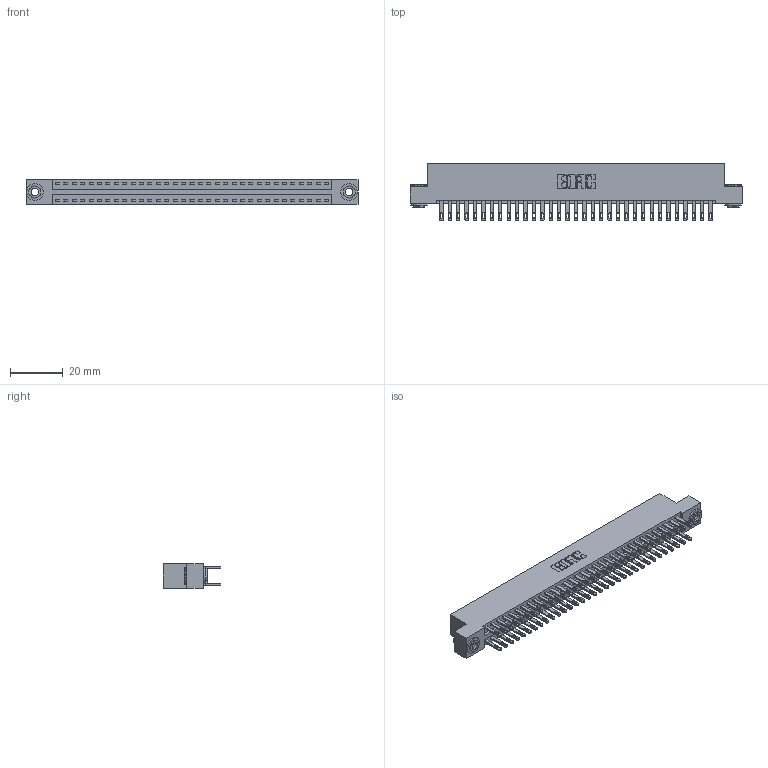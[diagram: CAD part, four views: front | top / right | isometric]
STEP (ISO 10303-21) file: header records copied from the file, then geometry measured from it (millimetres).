
FILE_DESCRIPTION (( 'STEP AP203' ), '1' );
FILE_NAME ('346-066-500-203.STEP', '2022-05-24T16:28:26', ( '' ), ( '' ), 'SwSTEP 2.0', 'SolidWorks 2020', '' );
FILE_SCHEMA (( 'CONFIG_CONTROL_DESIGN' ));
Length unit declared in the file: inch
Products named in the file (4): 346 Part_Flush Mounting Lugs - 0.156 Dia-TH; 345-250-002_345-250-002-102; 345-292-001_345-293-100; 346-066-500-203
Assembly tree (69 placements, depth 2):
  346-066-500-203
    346 Part_Flush Mounting Lugs - 0.156 Dia-TH
    345-292-001_345-293-100  x66
    345-250-002_345-250-002-102  x2
Bounding box: 125.35 x 21.84 x 9.4 mm (x, y, z)
Volume: 12356.2 mm3; surface area: 17782.4 mm2
Topology: 69 solids, 69 shells, 3342 faces, 10143 edges, 6758 vertices
Faces by surface type: plane 2014, cylinder 1320, cone 8
Entity records: 23744 total; most frequent: CARTESIAN_POINT 3905, ORIENTED_EDGE 3830, DIRECTION 3525, EDGE_CURVE 1915, LINE 1623, VECTOR 1623, VERTEX_POINT 1274, AXIS2_PLACEMENT_3D 951
